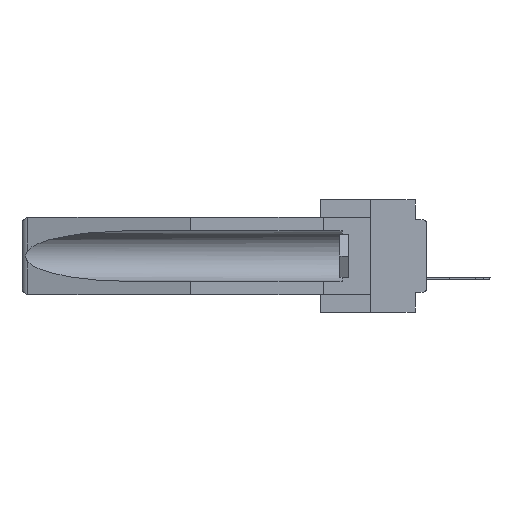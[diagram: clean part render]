
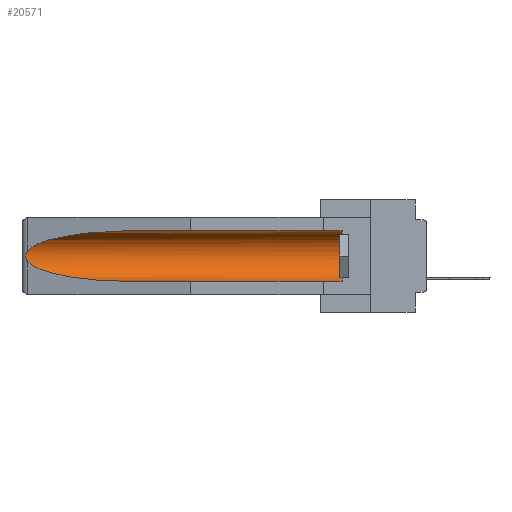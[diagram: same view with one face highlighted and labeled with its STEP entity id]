
A CAD part, left-side view. The second image highlights one B-rep face of the part: STEP entity #20571.
In plain terms, the highlighted cylindrical face has radius 2.857 mm (diameter 5.715 mm), a partial arc.
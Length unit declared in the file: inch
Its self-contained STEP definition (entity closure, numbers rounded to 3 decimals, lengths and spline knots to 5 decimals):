
#1738 = CARTESIAN_POINT ( 'NONE',  ( 0.26537, 1.52718, -0.14972 ) ) ;
#3359 = AXIS2_PLACEMENT_3D ( 'NONE', #11805, #16657, #33562 ) ;
#3681 = B_SPLINE_CURVE_WITH_KNOTS ( 'NONE', 3,
 ( #23044, #14762, #33821, #25371, #31298, #9200, #33985, #14939, #9545, #6859 ),
 .UNSPECIFIED., .F., .F.,
 ( 4, 2, 2, 2, 4 ),
 ( 0., 0.00029, 0.00058, 0.00087, 0.00117 ),
 .UNSPECIFIED. ) ;
#3892 = ORIENTED_EDGE ( 'NONE', *, *, #4867, .T. ) ;
#4867 = EDGE_CURVE ( 'NONE', #35088, #13482, #16397, .T. ) ;
#5058 = ORIENTED_EDGE ( 'NONE', *, *, #18193, .T. ) ;
#5886 = EDGE_CURVE ( 'NONE', #13761, #35088, #22871, .T. ) ;
#6859 = CARTESIAN_POINT ( 'NONE',  ( 0.26537, 1.52718, -0.19328 ) ) ;
#7098 = CARTESIAN_POINT ( 'NONE',  ( 0.155, 0.126, -0.284 ) ) ;
#7311 = AXIS2_PLACEMENT_3D ( 'NONE', #34557, #20389, #12097 ) ;
#7674 =( BOUNDED_CURVE ( )  B_SPLINE_CURVE ( 3, ( #33889, #11950, #25451, #17179 ),
 .UNSPECIFIED., .F., .T. ) 
 B_SPLINE_CURVE_WITH_KNOTS ( ( 4, 4 ),
 ( 0.1948, 1.5708 ),
 .UNSPECIFIED. ) 
 CURVE ( )  GEOMETRIC_REPRESENTATION_ITEM ( )  RATIONAL_B_SPLINE_CURVE ( ( 1., 0.848, 0.848, 1. ) ) 
 REPRESENTATION_ITEM ( '' )  );
#8182 = CARTESIAN_POINT ( 'NONE',  ( 0.21114, 1.30732, -0.059 ) ) ;
#8792 = VERTEX_POINT ( 'NONE', #16865 ) ;
#8996 = VERTEX_POINT ( 'NONE', #1738 ) ;
#9200 = CARTESIAN_POINT ( 'NONE',  ( 0.2675, 1.53308, -0.17534 ) ) ;
#9545 = CARTESIAN_POINT ( 'NONE',  ( 0.26597, 1.5296, -0.19026 ) ) ;
#10689 = CARTESIAN_POINT ( 'NONE',  ( 0.155, 1.07973, -0.059 ) ) ;
#11353 = CARTESIAN_POINT ( 'NONE',  ( 0.155, -0.30754, -0.059 ) ) ;
#11387 = ORIENTED_EDGE ( 'NONE', *, *, #21596, .T. ) ;
#11805 = CARTESIAN_POINT ( 'NONE',  ( 0.155, 0.126, -0.1715 ) ) ;
#11950 = CARTESIAN_POINT ( 'NONE',  ( 0.25451, 1.48313, -0.24835 ) ) ;
#12097 = DIRECTION ( 'NONE',  ( 0., 0., 1. ) ) ;
#13482 = VERTEX_POINT ( 'NONE', #26899 ) ;
#13761 = VERTEX_POINT ( 'NONE', #7098 ) ;
#14762 = CARTESIAN_POINT ( 'NONE',  ( 0.26597, 1.52961, -0.15275 ) ) ;
#14865 = EDGE_CURVE ( 'NONE', #27846, #8792, #7674, .T. ) ;
#14939 = CARTESIAN_POINT ( 'NONE',  ( 0.26655, 1.53094, -0.18657 ) ) ;
#16354 = VECTOR ( 'NONE', #20420, 39.37008 ) ;
#16397 = LINE ( 'NONE', #11353, #18918 ) ;
#16657 = DIRECTION ( 'NONE',  ( 0., -1., 0. ) ) ;
#16865 = CARTESIAN_POINT ( 'NONE',  ( 0.155, 1.07973, -0.284 ) ) ;
#17179 = CARTESIAN_POINT ( 'NONE',  ( 0.155, 1.07973, -0.284 ) ) ;
#17881 = CARTESIAN_POINT ( 'NONE',  ( 0.155, 0.126, -0.059 ) ) ;
#18193 = EDGE_CURVE ( 'NONE', #8996, #27846, #3681, .T. ) ;
#18474 =( BOUNDED_CURVE ( )  B_SPLINE_CURVE ( 3, ( #10689, #8182, #26882, #21670 ),
 .UNSPECIFIED., .F., .F. ) 
 B_SPLINE_CURVE_WITH_KNOTS ( ( 4, 4 ),
 ( 4.71239, 6.08839 ),
 .UNSPECIFIED. ) 
 CURVE ( )  GEOMETRIC_REPRESENTATION_ITEM ( )  RATIONAL_B_SPLINE_CURVE ( ( 1., 0.848, 0.848, 1. ) ) 
 REPRESENTATION_ITEM ( '' )  );
#18918 = VECTOR ( 'NONE', #29888, 39.37008 ) ;
#20389 = DIRECTION ( 'NONE',  ( 0., 1., 0. ) ) ;
#20420 = DIRECTION ( 'NONE',  ( 0., 1., 0. ) ) ;
#20571 = ADVANCED_FACE ( 'NONE', ( #26129 ), #23089, .F. ) ;
#21596 = EDGE_CURVE ( 'NONE', #13482, #8996, #18474, .T. ) ;
#21670 = CARTESIAN_POINT ( 'NONE',  ( 0.26537, 1.52718, -0.14972 ) ) ;
#22390 = ORIENTED_EDGE ( 'NONE', *, *, #34949, .F. ) ;
#22871 = CIRCLE ( 'NONE', #3359, 0.1125 ) ;
#23044 = CARTESIAN_POINT ( 'NONE',  ( 0.26537, 1.52718, -0.14972 ) ) ;
#23089 = CYLINDRICAL_SURFACE ( 'NONE', #7311, 0.1125 ) ;
#25371 = CARTESIAN_POINT ( 'NONE',  ( 0.2673, 1.5327, -0.16383 ) ) ;
#25451 = CARTESIAN_POINT ( 'NONE',  ( 0.21114, 1.30732, -0.284 ) ) ;
#25455 = LINE ( 'NONE', #30842, #16354 ) ;
#26129 = FACE_OUTER_BOUND ( 'NONE', #29742, .T. ) ;
#26882 = CARTESIAN_POINT ( 'NONE',  ( 0.25451, 1.48313, -0.09465 ) ) ;
#26899 = CARTESIAN_POINT ( 'NONE',  ( 0.155, 1.07973, -0.059 ) ) ;
#27028 = CARTESIAN_POINT ( 'NONE',  ( 0.26537, 1.52718, -0.19328 ) ) ;
#27846 = VERTEX_POINT ( 'NONE', #27028 ) ;
#29741 = ORIENTED_EDGE ( 'NONE', *, *, #5886, .T. ) ;
#29742 = EDGE_LOOP ( 'NONE', ( #11387, #5058, #31928, #22390, #29741, #3892 ) ) ;
#29888 = DIRECTION ( 'NONE',  ( 0., 1., 0. ) ) ;
#30842 = CARTESIAN_POINT ( 'NONE',  ( 0.155, -0.30754, -0.284 ) ) ;
#31298 = CARTESIAN_POINT ( 'NONE',  ( 0.2675, 1.53308, -0.16763 ) ) ;
#31928 = ORIENTED_EDGE ( 'NONE', *, *, #14865, .T. ) ;
#33562 = DIRECTION ( 'NONE',  ( 0., 0., 1. ) ) ;
#33821 = CARTESIAN_POINT ( 'NONE',  ( 0.26654, 1.53092, -0.15636 ) ) ;
#33889 = CARTESIAN_POINT ( 'NONE',  ( 0.26537, 1.52718, -0.19328 ) ) ;
#33985 = CARTESIAN_POINT ( 'NONE',  ( 0.2673, 1.53269, -0.17917 ) ) ;
#34557 = CARTESIAN_POINT ( 'NONE',  ( 0.155, -0.30754, -0.1715 ) ) ;
#34949 = EDGE_CURVE ( 'NONE', #13761, #8792, #25455, .T. ) ;
#35088 = VERTEX_POINT ( 'NONE', #17881 ) ;
